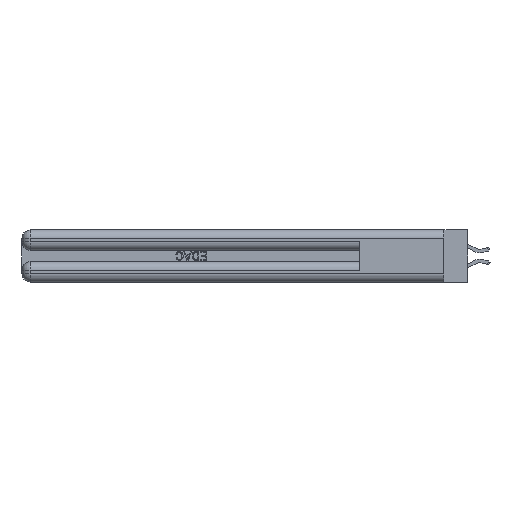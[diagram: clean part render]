
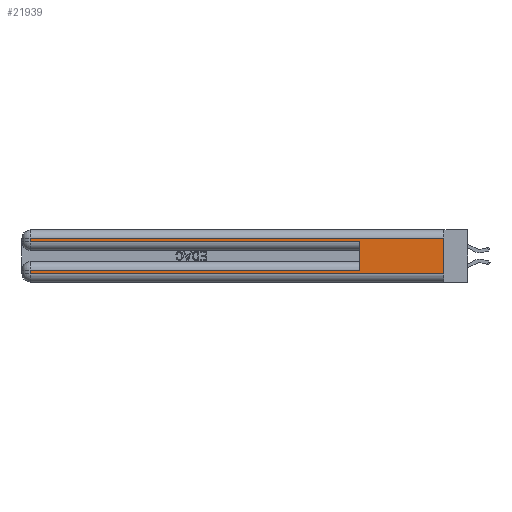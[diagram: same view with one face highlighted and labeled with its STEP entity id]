
A CAD part, left-side view. The second image highlights one B-rep face of the part: STEP entity #21939.
In plain terms, the highlighted planar face has unit normal (-1, 0, 0).
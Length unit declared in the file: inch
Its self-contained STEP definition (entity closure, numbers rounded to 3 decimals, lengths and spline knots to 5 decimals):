
#92 = DIRECTION ( 'NONE',  ( 0., -1., 0. ) ) ;
#908 = LINE ( 'NONE', #35166, #35660 ) ;
#1171 = DIRECTION ( 'NONE',  ( 0., 0., -1. ) ) ;
#2479 = CARTESIAN_POINT ( 'NONE',  ( 0., 0.6, 0.085 ) ) ;
#2865 = LINE ( 'NONE', #11483, #3770 ) ;
#2878 = VERTEX_POINT ( 'NONE', #31551 ) ;
#3045 = ORIENTED_EDGE ( 'NONE', *, *, #14896, .T. ) ;
#3089 = ORIENTED_EDGE ( 'NONE', *, *, #35507, .T. ) ;
#3592 = CARTESIAN_POINT ( 'NONE',  ( 0., 0., 0.06 ) ) ;
#3706 = LINE ( 'NONE', #8741, #8777 ) ;
#3770 = VECTOR ( 'NONE', #5203, 39.37008 ) ;
#3894 = DIRECTION ( 'NONE',  ( 0., 0., 1. ) ) ;
#4410 = EDGE_CURVE ( 'NONE', #13863, #20028, #908, .T. ) ;
#5203 = DIRECTION ( 'NONE',  ( 0., 1., 0. ) ) ;
#5631 = ORIENTED_EDGE ( 'NONE', *, *, #4410, .T. ) ;
#6720 = CARTESIAN_POINT ( 'NONE',  ( 0., 0.6, 0.145 ) ) ;
#8741 = CARTESIAN_POINT ( 'NONE',  ( 0., 0., 0.37 ) ) ;
#8777 = VECTOR ( 'NONE', #14586, 39.37008 ) ;
#8910 = DIRECTION ( 'NONE',  ( 0., 0., -1. ) ) ;
#9095 = VERTEX_POINT ( 'NONE', #32370 ) ;
#9475 = CARTESIAN_POINT ( 'NONE',  ( 0., 2.94, 0.085 ) ) ;
#10219 = VERTEX_POINT ( 'NONE', #11059 ) ;
#10287 = ORIENTED_EDGE ( 'NONE', *, *, #19264, .T. ) ;
#11049 = DIRECTION ( 'NONE',  ( 0., 0., -1. ) ) ;
#11059 = CARTESIAN_POINT ( 'NONE',  ( 0., 0.6, 0.285 ) ) ;
#11192 = VERTEX_POINT ( 'NONE', #27750 ) ;
#11436 = LINE ( 'NONE', #13069, #26554 ) ;
#11483 = CARTESIAN_POINT ( 'NONE',  ( 0., 0., 0.31 ) ) ;
#13069 = CARTESIAN_POINT ( 'NONE',  ( 0., 2.94, 0.37 ) ) ;
#13863 = VERTEX_POINT ( 'NONE', #24835 ) ;
#14439 = VERTEX_POINT ( 'NONE', #9475 ) ;
#14586 = DIRECTION ( 'NONE',  ( 0., 0., -1. ) ) ;
#14809 = DIRECTION ( 'NONE',  ( 0., 1., 0. ) ) ;
#14896 = EDGE_CURVE ( 'NONE', #31152, #14439, #28110, .T. ) ;
#16802 = DIRECTION ( 'NONE',  ( 1., 0., 0. ) ) ;
#16989 = AXIS2_PLACEMENT_3D ( 'NONE', #31261, #16802, #11049 ) ;
#18583 = EDGE_CURVE ( 'NONE', #2878, #10219, #24593, .T. ) ;
#18617 = EDGE_LOOP ( 'NONE', ( #28352, #3089, #35994, #36244, #35172, #3045, #10287, #5631 ) ) ;
#19264 = EDGE_CURVE ( 'NONE', #14439, #13863, #21425, .T. ) ;
#19546 = VECTOR ( 'NONE', #92, 39.37008 ) ;
#20028 = VERTEX_POINT ( 'NONE', #3592 ) ;
#21425 = LINE ( 'NONE', #26424, #28722 ) ;
#21939 = ADVANCED_FACE ( 'NONE', ( #32604 ), #28573, .F. ) ;
#22861 = EDGE_CURVE ( 'NONE', #11192, #20028, #3706, .T. ) ;
#24593 = LINE ( 'NONE', #37809, #19546 ) ;
#24835 = CARTESIAN_POINT ( 'NONE',  ( 0., 2.94, 0.06 ) ) ;
#25267 = LINE ( 'NONE', #6720, #35334 ) ;
#26424 = CARTESIAN_POINT ( 'NONE',  ( 0., 2.94, 0.37 ) ) ;
#26554 = VECTOR ( 'NONE', #1171, 39.37008 ) ;
#27750 = CARTESIAN_POINT ( 'NONE',  ( 0., 0., 0.31 ) ) ;
#28110 = LINE ( 'NONE', #32704, #37199 ) ;
#28352 = ORIENTED_EDGE ( 'NONE', *, *, #22861, .F. ) ;
#28558 = EDGE_CURVE ( 'NONE', #31152, #10219, #25267, .T. ) ;
#28573 = PLANE ( 'NONE',  #16989 ) ;
#28722 = VECTOR ( 'NONE', #8910, 39.37008 ) ;
#31152 = VERTEX_POINT ( 'NONE', #2479 ) ;
#31261 = CARTESIAN_POINT ( 'NONE',  ( 0., 0., 0.37 ) ) ;
#31551 = CARTESIAN_POINT ( 'NONE',  ( 0., 2.94, 0.285 ) ) ;
#32370 = CARTESIAN_POINT ( 'NONE',  ( 0., 2.94, 0.31 ) ) ;
#32604 = FACE_OUTER_BOUND ( 'NONE', #18617, .T. ) ;
#32704 = CARTESIAN_POINT ( 'NONE',  ( 0., 0., 0.085 ) ) ;
#34861 = DIRECTION ( 'NONE',  ( 0., -1., 0. ) ) ;
#35166 = CARTESIAN_POINT ( 'NONE',  ( 0., 0., 0.06 ) ) ;
#35172 = ORIENTED_EDGE ( 'NONE', *, *, #28558, .F. ) ;
#35334 = VECTOR ( 'NONE', #3894, 39.37008 ) ;
#35507 = EDGE_CURVE ( 'NONE', #11192, #9095, #2865, .T. ) ;
#35660 = VECTOR ( 'NONE', #34861, 39.37008 ) ;
#35994 = ORIENTED_EDGE ( 'NONE', *, *, #37869, .T. ) ;
#36244 = ORIENTED_EDGE ( 'NONE', *, *, #18583, .T. ) ;
#37199 = VECTOR ( 'NONE', #14809, 39.37008 ) ;
#37809 = CARTESIAN_POINT ( 'NONE',  ( 0., 0., 0.285 ) ) ;
#37869 = EDGE_CURVE ( 'NONE', #9095, #2878, #11436, .T. ) ;
